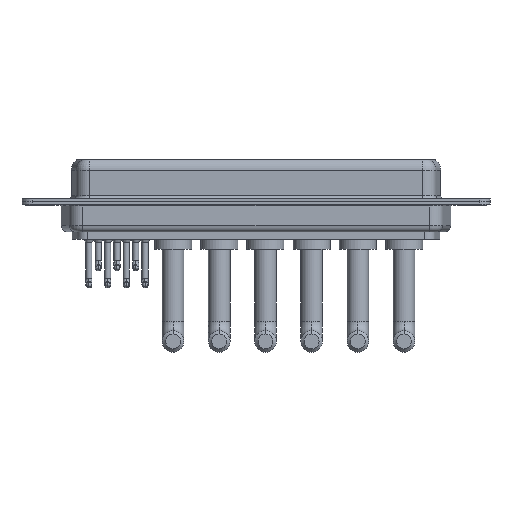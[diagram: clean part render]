
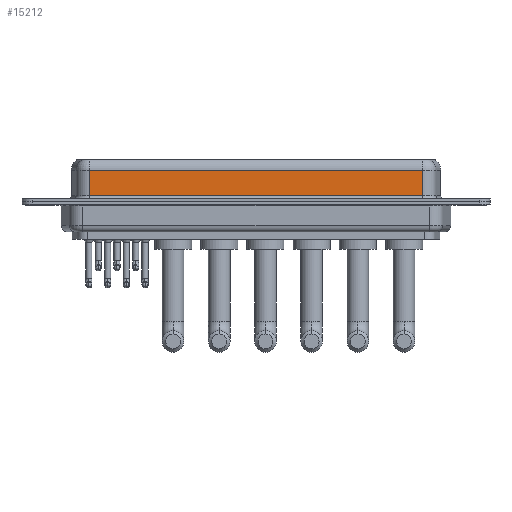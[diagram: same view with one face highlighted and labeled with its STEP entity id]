
A CAD part, front view. The second image highlights one B-rep face of the part: STEP entity #15212.
In plain terms, the highlighted planar face has unit normal (0, -1, 0).
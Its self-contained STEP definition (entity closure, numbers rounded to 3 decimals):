
#20 = EDGE_LOOP ( 'NONE', ( #14571, #3594, #2192, #15267 ) ) ;
#495 = VERTEX_POINT ( 'NONE', #9946 ) ;
#674 = VECTOR ( 'NONE', #14551, 1000. ) ;
#692 = CARTESIAN_POINT ( 'NONE',  ( 56.462, -3.95, 6.4 ) ) ;
#758 = EDGE_CURVE ( 'NONE', #495, #888, #2896, .T. ) ;
#888 = VERTEX_POINT ( 'NONE', #12422 ) ;
#1045 = VERTEX_POINT ( 'NONE', #13313 ) ;
#1062 = LINE ( 'NONE', #8829, #10487 ) ;
#2116 = VECTOR ( 'NONE', #13399, 1000. ) ;
#2192 = ORIENTED_EDGE ( 'NONE', *, *, #6418, .T. ) ;
#2422 = DIRECTION ( 'NONE',  ( 0., 0., -1. ) ) ;
#2896 = LINE ( 'NONE', #10734, #13865 ) ;
#2980 = EDGE_CURVE ( 'NONE', #1045, #16113, #3284, .T. ) ;
#3284 = LINE ( 'NONE', #6000, #674 ) ;
#3418 = DIRECTION ( 'NONE',  ( 0., 1., 0. ) ) ;
#3499 = AXIS2_PLACEMENT_3D ( 'NONE', #692, #3418, #9738 ) ;
#3594 = ORIENTED_EDGE ( 'NONE', *, *, #2980, .T. ) ;
#4394 = LINE ( 'NONE', #13146, #2116 ) ;
#6000 = CARTESIAN_POINT ( 'NONE',  ( 56.462, -3.95, 4.65 ) ) ;
#6418 = EDGE_CURVE ( 'NONE', #16113, #495, #4394, .T. ) ;
#8829 = CARTESIAN_POINT ( 'NONE',  ( 56.462, -3.95, 6.4 ) ) ;
#9738 = DIRECTION ( 'NONE',  ( 0., 0., 1. ) ) ;
#9946 = CARTESIAN_POINT ( 'NONE',  ( 7.038, -3.95, 0.9 ) ) ;
#10093 = CARTESIAN_POINT ( 'NONE',  ( 7.038, -3.95, 4.65 ) ) ;
#10487 = VECTOR ( 'NONE', #2422, 1000. ) ;
#10734 = CARTESIAN_POINT ( 'NONE',  ( 56.462, -3.95, 0.9 ) ) ;
#10997 = PLANE ( 'NONE',  #3499 ) ;
#12079 = DIRECTION ( 'NONE',  ( 1., 0., 0. ) ) ;
#12175 = FACE_OUTER_BOUND ( 'NONE', #20, .T. ) ;
#12422 = CARTESIAN_POINT ( 'NONE',  ( 56.462, -3.95, 0.9 ) ) ;
#13146 = CARTESIAN_POINT ( 'NONE',  ( 7.038, -3.95, 6.4 ) ) ;
#13313 = CARTESIAN_POINT ( 'NONE',  ( 56.462, -3.95, 4.65 ) ) ;
#13399 = DIRECTION ( 'NONE',  ( 0., 0., -1. ) ) ;
#13865 = VECTOR ( 'NONE', #12079, 1000. ) ;
#14551 = DIRECTION ( 'NONE',  ( -1., 0., 0. ) ) ;
#14571 = ORIENTED_EDGE ( 'NONE', *, *, #15026, .F. ) ;
#15026 = EDGE_CURVE ( 'NONE', #1045, #888, #1062, .T. ) ;
#15212 = ADVANCED_FACE ( 'NONE', ( #12175 ), #10997, .F. ) ;
#15267 = ORIENTED_EDGE ( 'NONE', *, *, #758, .T. ) ;
#16113 = VERTEX_POINT ( 'NONE', #10093 ) ;
